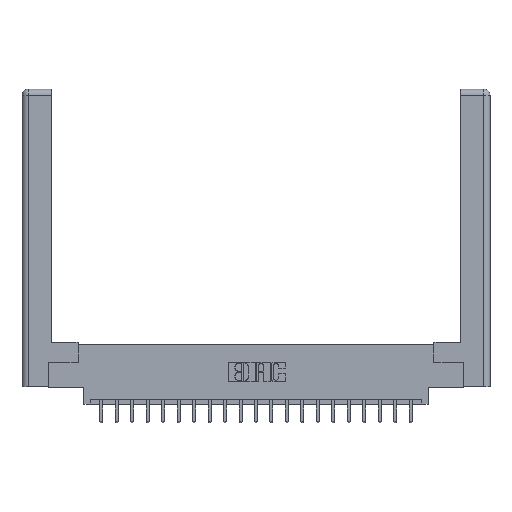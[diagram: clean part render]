
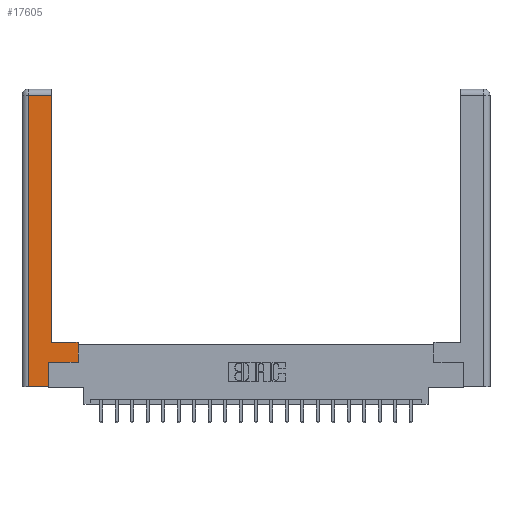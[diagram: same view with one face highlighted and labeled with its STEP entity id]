
A CAD part, top view. The second image highlights one B-rep face of the part: STEP entity #17605.
In plain terms, the highlighted planar face has unit normal (0, 0, 1).
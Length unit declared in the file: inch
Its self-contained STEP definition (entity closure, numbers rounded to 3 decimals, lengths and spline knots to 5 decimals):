
#444 = DIRECTION ( 'NONE',  ( 0., 0., -1. ) ) ;
#1218 = DIRECTION ( 'NONE',  ( 1., 0., 0. ) ) ;
#1633 = VECTOR ( 'NONE', #18266, 39.37008 ) ;
#1764 = VECTOR ( 'NONE', #18990, 39.37008 ) ;
#1817 = DIRECTION ( 'NONE',  ( 0., 1., 0. ) ) ;
#1894 = LINE ( 'NONE', #15084, #1633 ) ;
#2051 = FACE_OUTER_BOUND ( 'NONE', #7657, .T. ) ;
#3623 = PLANE ( 'NONE',  #7981 ) ;
#3851 = VERTEX_POINT ( 'NONE', #5391 ) ;
#3868 = CARTESIAN_POINT ( 'NONE',  ( 0.265, 0.245, 0. ) ) ;
#4695 = DIRECTION ( 'NONE',  ( -1., 0., 0. ) ) ;
#4797 = DIRECTION ( 'NONE',  ( 0., -1., 0. ) ) ;
#4885 = ORIENTED_EDGE ( 'NONE', *, *, #8137, .T. ) ;
#5060 = CARTESIAN_POINT ( 'NONE',  ( 0.565, 0.45, 0. ) ) ;
#5281 = EDGE_CURVE ( 'NONE', #14952, #18718, #7105, .T. ) ;
#5391 = CARTESIAN_POINT ( 'NONE',  ( 0.0615, 2.94, 0. ) ) ;
#5827 = LINE ( 'NONE', #18102, #11075 ) ;
#6178 = VECTOR ( 'NONE', #4797, 39.37008 ) ;
#6735 = ORIENTED_EDGE ( 'NONE', *, *, #12683, .T. ) ;
#6758 = EDGE_CURVE ( 'NONE', #21270, #19864, #15459, .T. ) ;
#7105 = LINE ( 'NONE', #19795, #10785 ) ;
#7261 = CARTESIAN_POINT ( 'NONE',  ( 0.565, 0.45, 0. ) ) ;
#7657 = EDGE_LOOP ( 'NONE', ( #15652, #4885, #10112, #21677, #8704, #16702, #17546, #6735 ) ) ;
#7981 = AXIS2_PLACEMENT_3D ( 'NONE', #20622, #444, #20549 ) ;
#8002 = EDGE_CURVE ( 'NONE', #3851, #14231, #9080, .T. ) ;
#8137 = EDGE_CURVE ( 'NONE', #18718, #3851, #19382, .T. ) ;
#8330 = CARTESIAN_POINT ( 'NONE',  ( 0.0615, 0., 0. ) ) ;
#8704 = ORIENTED_EDGE ( 'NONE', *, *, #6758, .T. ) ;
#9080 = LINE ( 'NONE', #8330, #6178 ) ;
#9602 = EDGE_CURVE ( 'NONE', #14231, #21270, #1894, .T. ) ;
#9857 = VECTOR ( 'NONE', #11979, 39.37008 ) ;
#10112 = ORIENTED_EDGE ( 'NONE', *, *, #8002, .T. ) ;
#10785 = VECTOR ( 'NONE', #12432, 39.37008 ) ;
#11075 = VECTOR ( 'NONE', #4695, 39.37008 ) ;
#11615 = EDGE_CURVE ( 'NONE', #17672, #13502, #11653, .T. ) ;
#11653 = LINE ( 'NONE', #5060, #16175 ) ;
#11979 = DIRECTION ( 'NONE',  ( -1., 0., 0. ) ) ;
#12432 = DIRECTION ( 'NONE',  ( 0., 1., 0. ) ) ;
#12683 = EDGE_CURVE ( 'NONE', #13502, #14952, #5827, .T. ) ;
#13502 = VERTEX_POINT ( 'NONE', #7261 ) ;
#13648 = CARTESIAN_POINT ( 'NONE',  ( 0.295, 2.94, 0. ) ) ;
#14061 = VECTOR ( 'NONE', #1218, 39.37008 ) ;
#14231 = VERTEX_POINT ( 'NONE', #19939 ) ;
#14289 = CARTESIAN_POINT ( 'NONE',  ( 0.265, 0.245, 0. ) ) ;
#14340 = CARTESIAN_POINT ( 'NONE',  ( 0.265, 0., 0. ) ) ;
#14952 = VERTEX_POINT ( 'NONE', #21254 ) ;
#15084 = CARTESIAN_POINT ( 'NONE',  ( 0.265, 0., 0. ) ) ;
#15459 = LINE ( 'NONE', #3868, #1764 ) ;
#15652 = ORIENTED_EDGE ( 'NONE', *, *, #5281, .T. ) ;
#16175 = VECTOR ( 'NONE', #1817, 39.37008 ) ;
#16702 = ORIENTED_EDGE ( 'NONE', *, *, #17299, .T. ) ;
#16956 = CARTESIAN_POINT ( 'NONE',  ( 0.0615, 2.94, 0. ) ) ;
#17299 = EDGE_CURVE ( 'NONE', #19864, #17672, #21258, .T. ) ;
#17546 = ORIENTED_EDGE ( 'NONE', *, *, #11615, .T. ) ;
#17605 = ADVANCED_FACE ( 'NONE', ( #2051 ), #3623, .F. ) ;
#17672 = VERTEX_POINT ( 'NONE', #17684 ) ;
#17684 = CARTESIAN_POINT ( 'NONE',  ( 0.565, 0.245, 0. ) ) ;
#18102 = CARTESIAN_POINT ( 'NONE',  ( 0.295, 0.45, 0. ) ) ;
#18266 = DIRECTION ( 'NONE',  ( 1., 0., 0. ) ) ;
#18718 = VERTEX_POINT ( 'NONE', #13648 ) ;
#18990 = DIRECTION ( 'NONE',  ( 0., 1., 0. ) ) ;
#19382 = LINE ( 'NONE', #16956, #9857 ) ;
#19535 = CARTESIAN_POINT ( 'NONE',  ( 0.565, 0.245, 0. ) ) ;
#19795 = CARTESIAN_POINT ( 'NONE',  ( 0.295, 3., 0. ) ) ;
#19864 = VERTEX_POINT ( 'NONE', #14289 ) ;
#19939 = CARTESIAN_POINT ( 'NONE',  ( 0.0615, 0., 0. ) ) ;
#20549 = DIRECTION ( 'NONE',  ( -1., 0., 0. ) ) ;
#20622 = CARTESIAN_POINT ( 'NONE',  ( 0., 0., 0. ) ) ;
#21254 = CARTESIAN_POINT ( 'NONE',  ( 0.295, 0.45, 0. ) ) ;
#21258 = LINE ( 'NONE', #19535, #14061 ) ;
#21270 = VERTEX_POINT ( 'NONE', #14340 ) ;
#21677 = ORIENTED_EDGE ( 'NONE', *, *, #9602, .T. ) ;
